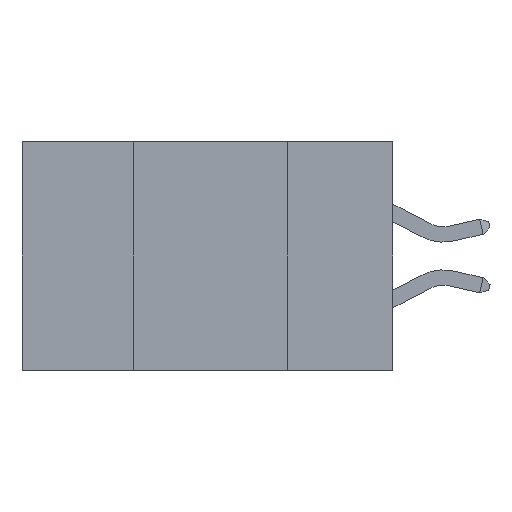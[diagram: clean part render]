
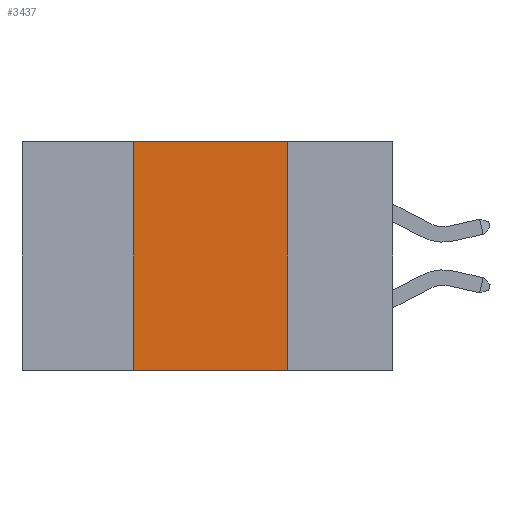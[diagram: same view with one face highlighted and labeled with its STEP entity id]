
A CAD part, left-side view. The second image highlights one B-rep face of the part: STEP entity #3437.
In plain terms, the highlighted planar face has unit normal (-1, 0, 0).
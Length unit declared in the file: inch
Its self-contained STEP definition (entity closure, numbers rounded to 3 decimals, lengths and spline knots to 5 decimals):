
#94 = ORIENTED_EDGE ( 'NONE', *, *, #18274, .F. ) ;
#510 = EDGE_CURVE ( 'NONE', #18602, #19742, #16872, .T. ) ;
#2020 = VERTEX_POINT ( 'NONE', #18343 ) ;
#3437 = ADVANCED_FACE ( 'NONE', ( #13961 ), #7028, .F. ) ;
#4140 = CARTESIAN_POINT ( 'NONE',  ( 0., 0.17, -0.37 ) ) ;
#4716 = DIRECTION ( 'NONE',  ( 0., 0., 1. ) ) ;
#5104 = DIRECTION ( 'NONE',  ( 0., 0., -1. ) ) ;
#5661 = CARTESIAN_POINT ( 'NONE',  ( 0., 0.6, 0. ) ) ;
#6324 = EDGE_LOOP ( 'NONE', ( #7563, #94, #9152, #15306 ) ) ;
#6499 = LINE ( 'NONE', #16511, #8188 ) ;
#6771 = DIRECTION ( 'NONE',  ( 0., -1., 0. ) ) ;
#7028 = PLANE ( 'NONE',  #19578 ) ;
#7338 = EDGE_CURVE ( 'NONE', #2020, #8251, #6499, .T. ) ;
#7563 = ORIENTED_EDGE ( 'NONE', *, *, #7338, .F. ) ;
#7589 = DIRECTION ( 'NONE',  ( 0., 0., -1. ) ) ;
#8188 = VECTOR ( 'NONE', #7589, 39.37008 ) ;
#8251 = VERTEX_POINT ( 'NONE', #4140 ) ;
#9152 = ORIENTED_EDGE ( 'NONE', *, *, #510, .F. ) ;
#9367 = LINE ( 'NONE', #5661, #20711 ) ;
#9784 = VECTOR ( 'NONE', #6771, 39.37008 ) ;
#10572 = CARTESIAN_POINT ( 'NONE',  ( 0., 0.6, 0. ) ) ;
#13961 = FACE_OUTER_BOUND ( 'NONE', #6324, .T. ) ;
#15306 = ORIENTED_EDGE ( 'NONE', *, *, #21986, .T. ) ;
#15608 = CARTESIAN_POINT ( 'NONE',  ( 0., 0.6, -0.37 ) ) ;
#15754 = CARTESIAN_POINT ( 'NONE',  ( 0., 0.42, -0.37 ) ) ;
#16511 = CARTESIAN_POINT ( 'NONE',  ( 0., 0.17, 0. ) ) ;
#16800 = DIRECTION ( 'NONE',  ( 0., -1., 0. ) ) ;
#16872 = LINE ( 'NONE', #19242, #17737 ) ;
#17737 = VECTOR ( 'NONE', #4716, 39.37008 ) ;
#18274 = EDGE_CURVE ( 'NONE', #19742, #2020, #9367, .T. ) ;
#18343 = CARTESIAN_POINT ( 'NONE',  ( 0., 0.17, 0. ) ) ;
#18602 = VERTEX_POINT ( 'NONE', #15754 ) ;
#19242 = CARTESIAN_POINT ( 'NONE',  ( 0., 0.42, 0. ) ) ;
#19578 = AXIS2_PLACEMENT_3D ( 'NONE', #10572, #21411, #5104 ) ;
#19742 = VERTEX_POINT ( 'NONE', #22469 ) ;
#20711 = VECTOR ( 'NONE', #16800, 39.37008 ) ;
#21411 = DIRECTION ( 'NONE',  ( 1., 0., 0. ) ) ;
#21950 = LINE ( 'NONE', #15608, #9784 ) ;
#21986 = EDGE_CURVE ( 'NONE', #18602, #8251, #21950, .T. ) ;
#22469 = CARTESIAN_POINT ( 'NONE',  ( 0., 0.42, 0. ) ) ;
